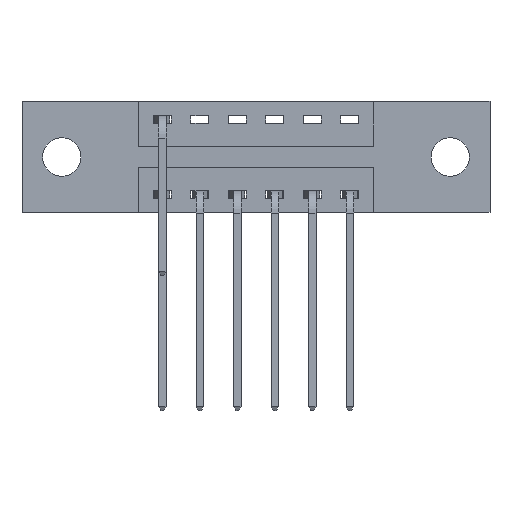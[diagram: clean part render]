
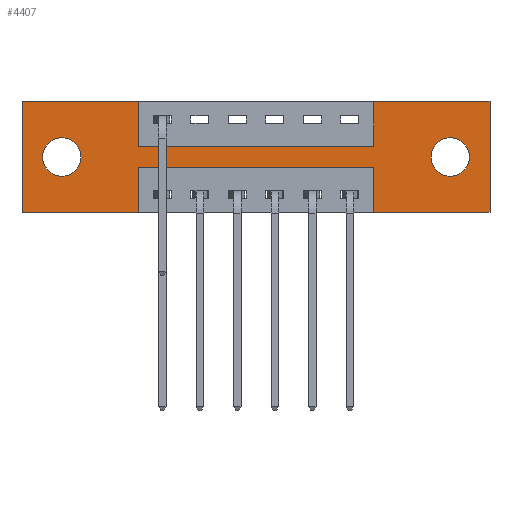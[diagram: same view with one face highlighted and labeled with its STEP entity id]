
A CAD part, front view. The second image highlights one B-rep face of the part: STEP entity #4407.
In plain terms, the highlighted planar face has unit normal (0, -1, 0).
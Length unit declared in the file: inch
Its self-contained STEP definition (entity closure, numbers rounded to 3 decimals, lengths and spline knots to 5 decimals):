
#35 = VECTOR ( 'NONE', #1929, 39.37008 ) ;
#183 = VERTEX_POINT ( 'NONE', #6372 ) ;
#195 = CARTESIAN_POINT ( 'NONE',  ( 0.1325, 0., -0.121 ) ) ;
#269 = CARTESIAN_POINT ( 'NONE',  ( 0., 0., 0. ) ) ;
#292 = LINE ( 'NONE', #3707, #4562 ) ;
#306 = LINE ( 'NONE', #2538, #4321 ) ;
#589 = VECTOR ( 'NONE', #6470, 39.37008 ) ;
#642 = DIRECTION ( 'NONE',  ( -1., 0., 0. ) ) ;
#678 = CARTESIAN_POINT ( 'NONE',  ( 0.1325, 0., -0.249 ) ) ;
#759 = VECTOR ( 'NONE', #4111, 39.37008 ) ;
#803 = EDGE_CURVE ( 'NONE', #2484, #2592, #8402, .T. ) ;
#855 = DIRECTION ( 'NONE',  ( 0., 0., -1. ) ) ;
#1016 = AXIS2_PLACEMENT_3D ( 'NONE', #7926, #3055, #8718 ) ;
#1052 = VERTEX_POINT ( 'NONE', #195 ) ;
#1143 = EDGE_CURVE ( 'NONE', #7523, #8817, #306, .T. ) ;
#1165 = CARTESIAN_POINT ( 'NONE',  ( 0., 0., 0. ) ) ;
#1189 = CARTESIAN_POINT ( 'NONE',  ( 0., 0., -0.37 ) ) ;
#1305 = CARTESIAN_POINT ( 'NONE',  ( 1.1725, 0., -0.37 ) ) ;
#1366 = CARTESIAN_POINT ( 'NONE',  ( 1.56, 0., -0.37 ) ) ;
#1513 = EDGE_CURVE ( 'NONE', #8817, #3259, #3452, .T. ) ;
#1577 = CARTESIAN_POINT ( 'NONE',  ( 0.3875, 0., 0. ) ) ;
#1594 = PLANE ( 'NONE',  #1831 ) ;
#1831 = AXIS2_PLACEMENT_3D ( 'NONE', #10384, #5642, #855 ) ;
#1929 = DIRECTION ( 'NONE',  ( 0., 0., 1. ) ) ;
#2026 = EDGE_CURVE ( 'NONE', #6232, #7523, #6995, .T. ) ;
#2185 = VERTEX_POINT ( 'NONE', #3243 ) ;
#2328 = DIRECTION ( 'NONE',  ( 0., 1., 0. ) ) ;
#2346 = DIRECTION ( 'NONE',  ( -1., 0., 0. ) ) ;
#2442 = CARTESIAN_POINT ( 'NONE',  ( 0.3875, 0., -0.37 ) ) ;
#2484 = VERTEX_POINT ( 'NONE', #4684 ) ;
#2494 = EDGE_CURVE ( 'NONE', #7494, #183, #2781, .T. ) ;
#2538 = CARTESIAN_POINT ( 'NONE',  ( 1.1725, 0., 0. ) ) ;
#2592 = VERTEX_POINT ( 'NONE', #1577 ) ;
#2781 = LINE ( 'NONE', #5805, #6875 ) ;
#2788 = VERTEX_POINT ( 'NONE', #1305 ) ;
#3055 = DIRECTION ( 'NONE',  ( 0., 1., 0. ) ) ;
#3155 = VERTEX_POINT ( 'NONE', #2442 ) ;
#3243 = CARTESIAN_POINT ( 'NONE',  ( 1.4275, 0., -0.249 ) ) ;
#3259 = VERTEX_POINT ( 'NONE', #6530 ) ;
#3341 = VECTOR ( 'NONE', #8262, 39.37008 ) ;
#3426 = EDGE_CURVE ( 'NONE', #5576, #2185, #4245, .T. ) ;
#3452 = LINE ( 'NONE', #5753, #5315 ) ;
#3658 = DIRECTION ( 'NONE',  ( 0., 1., 0. ) ) ;
#3664 = CARTESIAN_POINT ( 'NONE',  ( 0.3875, 0., 0. ) ) ;
#3707 = CARTESIAN_POINT ( 'NONE',  ( 1.56, 0., 0. ) ) ;
#3729 = LINE ( 'NONE', #6488, #4228 ) ;
#3736 = CARTESIAN_POINT ( 'NONE',  ( 0.3875, 0., -0.15 ) ) ;
#3824 = EDGE_CURVE ( 'NONE', #2788, #7494, #7192, .T. ) ;
#3981 = FACE_BOUND ( 'NONE', #9527, .T. ) ;
#4024 = DIRECTION ( 'NONE',  ( 0., 0., -1. ) ) ;
#4037 = VERTEX_POINT ( 'NONE', #1189 ) ;
#4074 = EDGE_CURVE ( 'NONE', #2592, #6232, #9166, .T. ) ;
#4111 = DIRECTION ( 'NONE',  ( 0., 0., 1. ) ) ;
#4228 = VECTOR ( 'NONE', #2346, 39.37008 ) ;
#4245 = CIRCLE ( 'NONE', #9463, 0.064 ) ;
#4288 = CARTESIAN_POINT ( 'NONE',  ( 1.4275, 0., -0.185 ) ) ;
#4321 = VECTOR ( 'NONE', #9942, 39.37008 ) ;
#4407 = ADVANCED_FACE ( 'NONE', ( #3981, #10098, #5903 ), #1594, .T. ) ;
#4417 = EDGE_CURVE ( 'NONE', #3155, #4037, #3729, .T. ) ;
#4435 = CARTESIAN_POINT ( 'NONE',  ( 1.1725, 0., -0.37 ) ) ;
#4441 = CARTESIAN_POINT ( 'NONE',  ( 1.4275, 0., -0.121 ) ) ;
#4452 = DIRECTION ( 'NONE',  ( -1., 0., 0. ) ) ;
#4465 = DIRECTION ( 'NONE',  ( 0., 0., -1. ) ) ;
#4562 = VECTOR ( 'NONE', #5304, 39.37008 ) ;
#4602 = VECTOR ( 'NONE', #4465, 39.37008 ) ;
#4684 = CARTESIAN_POINT ( 'NONE',  ( 0., 0., 0. ) ) ;
#4971 = CARTESIAN_POINT ( 'NONE',  ( 1.4275, 0., -0.185 ) ) ;
#5016 = EDGE_CURVE ( 'NONE', #7517, #2788, #7546, .T. ) ;
#5084 = DIRECTION ( 'NONE',  ( 0., 0., -1. ) ) ;
#5170 = VECTOR ( 'NONE', #6010, 39.37008 ) ;
#5304 = DIRECTION ( 'NONE',  ( 0., 0., -1. ) ) ;
#5313 = CARTESIAN_POINT ( 'NONE',  ( 1.1725, 0., -0.22 ) ) ;
#5315 = VECTOR ( 'NONE', #6319, 39.37008 ) ;
#5409 = CIRCLE ( 'NONE', #1016, 0.064 ) ;
#5576 = VERTEX_POINT ( 'NONE', #4441 ) ;
#5577 = AXIS2_PLACEMENT_3D ( 'NONE', #4288, #9900, #5084 ) ;
#5642 = DIRECTION ( 'NONE',  ( 0., -1., 0. ) ) ;
#5753 = CARTESIAN_POINT ( 'NONE',  ( 0., 0., 0. ) ) ;
#5805 = CARTESIAN_POINT ( 'NONE',  ( 0.3875, 0., -0.22 ) ) ;
#5903 = FACE_OUTER_BOUND ( 'NONE', #6173, .T. ) ;
#6010 = DIRECTION ( 'NONE',  ( 0., 0., -1. ) ) ;
#6173 = EDGE_LOOP ( 'NONE', ( #8891, #8925, #9052, #9167, #9264, #9378, #9435, #10171, #10259, #9940, #10354, #9753 ) ) ;
#6183 = EDGE_CURVE ( 'NONE', #3259, #7517, #292, .T. ) ;
#6232 = VERTEX_POINT ( 'NONE', #3736 ) ;
#6319 = DIRECTION ( 'NONE',  ( 1., 0., 0. ) ) ;
#6372 = CARTESIAN_POINT ( 'NONE',  ( 0.3875, 0., -0.22 ) ) ;
#6470 = DIRECTION ( 'NONE',  ( 1., 0., 0. ) ) ;
#6488 = CARTESIAN_POINT ( 'NONE',  ( 0., 0., -0.37 ) ) ;
#6530 = CARTESIAN_POINT ( 'NONE',  ( 1.56, 0., 0. ) ) ;
#6825 = CARTESIAN_POINT ( 'NONE',  ( 0.3875, 0., -0.37 ) ) ;
#6873 = EDGE_CURVE ( 'NONE', #183, #3155, #7392, .T. ) ;
#6875 = VECTOR ( 'NONE', #4452, 39.37008 ) ;
#6995 = LINE ( 'NONE', #7327, #589 ) ;
#7075 = CARTESIAN_POINT ( 'NONE',  ( 0., 0., -0.37 ) ) ;
#7192 = LINE ( 'NONE', #4435, #759 ) ;
#7242 = CARTESIAN_POINT ( 'NONE',  ( 0.1325, 0., -0.185 ) ) ;
#7300 = VECTOR ( 'NONE', #642, 39.37008 ) ;
#7327 = CARTESIAN_POINT ( 'NONE',  ( 0.3875, 0., -0.15 ) ) ;
#7387 = EDGE_LOOP ( 'NONE', ( #8739, #8805 ) ) ;
#7392 = LINE ( 'NONE', #6825, #5170 ) ;
#7494 = VERTEX_POINT ( 'NONE', #5313 ) ;
#7517 = VERTEX_POINT ( 'NONE', #1366 ) ;
#7523 = VERTEX_POINT ( 'NONE', #7829 ) ;
#7546 = LINE ( 'NONE', #7075, #7300 ) ;
#7829 = CARTESIAN_POINT ( 'NONE',  ( 1.1725, 0., -0.15 ) ) ;
#7908 = CIRCLE ( 'NONE', #5577, 0.064 ) ;
#7926 = CARTESIAN_POINT ( 'NONE',  ( 0.1325, 0., -0.185 ) ) ;
#8039 = DIRECTION ( 'NONE',  ( 0., 0., 1. ) ) ;
#8262 = DIRECTION ( 'NONE',  ( 1., 0., 0. ) ) ;
#8402 = LINE ( 'NONE', #269, #3341 ) ;
#8426 = EDGE_CURVE ( 'NONE', #1052, #9013, #5409, .T. ) ;
#8648 = ORIENTED_EDGE ( 'NONE', *, *, #3426, .T. ) ;
#8702 = ORIENTED_EDGE ( 'NONE', *, *, #10029, .T. ) ;
#8718 = DIRECTION ( 'NONE',  ( 0., 0., 1. ) ) ;
#8739 = ORIENTED_EDGE ( 'NONE', *, *, #8426, .T. ) ;
#8805 = ORIENTED_EDGE ( 'NONE', *, *, #9752, .T. ) ;
#8817 = VERTEX_POINT ( 'NONE', #9894 ) ;
#8891 = ORIENTED_EDGE ( 'NONE', *, *, #6873, .F. ) ;
#8925 = ORIENTED_EDGE ( 'NONE', *, *, #2494, .F. ) ;
#9013 = VERTEX_POINT ( 'NONE', #678 ) ;
#9026 = AXIS2_PLACEMENT_3D ( 'NONE', #7242, #2328, #8039 ) ;
#9052 = ORIENTED_EDGE ( 'NONE', *, *, #3824, .F. ) ;
#9158 = LINE ( 'NONE', #1165, #35 ) ;
#9166 = LINE ( 'NONE', #3664, #4602 ) ;
#9167 = ORIENTED_EDGE ( 'NONE', *, *, #5016, .F. ) ;
#9264 = ORIENTED_EDGE ( 'NONE', *, *, #6183, .F. ) ;
#9378 = ORIENTED_EDGE ( 'NONE', *, *, #1513, .F. ) ;
#9435 = ORIENTED_EDGE ( 'NONE', *, *, #1143, .F. ) ;
#9463 = AXIS2_PLACEMENT_3D ( 'NONE', #4971, #3658, #4024 ) ;
#9483 = EDGE_CURVE ( 'NONE', #4037, #2484, #9158, .T. ) ;
#9527 = EDGE_LOOP ( 'NONE', ( #8648, #8702 ) ) ;
#9752 = EDGE_CURVE ( 'NONE', #9013, #1052, #10332, .T. ) ;
#9753 = ORIENTED_EDGE ( 'NONE', *, *, #4417, .F. ) ;
#9894 = CARTESIAN_POINT ( 'NONE',  ( 1.1725, 0., 0. ) ) ;
#9900 = DIRECTION ( 'NONE',  ( 0., 1., 0. ) ) ;
#9940 = ORIENTED_EDGE ( 'NONE', *, *, #803, .F. ) ;
#9942 = DIRECTION ( 'NONE',  ( 0., 0., 1. ) ) ;
#10029 = EDGE_CURVE ( 'NONE', #2185, #5576, #7908, .T. ) ;
#10098 = FACE_BOUND ( 'NONE', #7387, .T. ) ;
#10171 = ORIENTED_EDGE ( 'NONE', *, *, #2026, .F. ) ;
#10259 = ORIENTED_EDGE ( 'NONE', *, *, #4074, .F. ) ;
#10332 = CIRCLE ( 'NONE', #9026, 0.064 ) ;
#10354 = ORIENTED_EDGE ( 'NONE', *, *, #9483, .F. ) ;
#10384 = CARTESIAN_POINT ( 'NONE',  ( 0., 0., -0.37 ) ) ;
